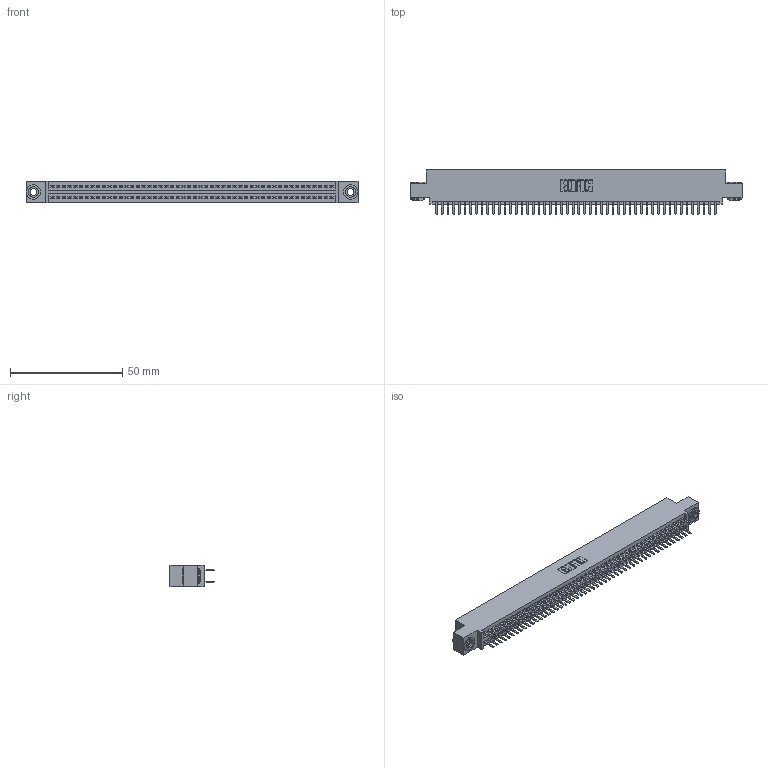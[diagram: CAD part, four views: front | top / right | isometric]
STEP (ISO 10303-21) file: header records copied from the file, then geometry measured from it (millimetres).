
FILE_DESCRIPTION (( 'STEP AP203' ), '1' );
FILE_NAME ('345-100-520-503.STEP', '2018-10-05T13:06:23', ( '' ), ( '' ), 'SwSTEP 2.0', 'SolidWorks 2016', '' );
FILE_SCHEMA (( 'CONFIG_CONTROL_DESIGN' ));
Length unit declared in the file: inch
Products named in the file (4): 345-250-002_345-250-002-102; 345 Part_0.110 Offset - 0.156 Dia-TH; 345-292-001_345-293-120; 345-100-520-503
Assembly tree (103 placements, depth 2):
  345-100-520-503
    345 Part_0.110 Offset - 0.156 Dia-TH
    345-292-001_345-293-120  x100
    345-250-002_345-250-002-102  x2
Bounding box: 148.21 x 19.68 x 9.4 mm (x, y, z)
Volume: 14373.5 mm3; surface area: 21605.6 mm2
Topology: 103 solids, 103 shells, 5568 faces, 16129 edges, 10482 vertices
Faces by surface type: plane 3594, cylinder 1966, cone 8
Entity records: 39050 total; most frequent: CARTESIAN_POINT 6527, ORIENTED_EDGE 6442, DIRECTION 5763, EDGE_CURVE 3221, LINE 2861, VECTOR 2861, VERTEX_POINT 2142, AXIS2_PLACEMENT_3D 1451
